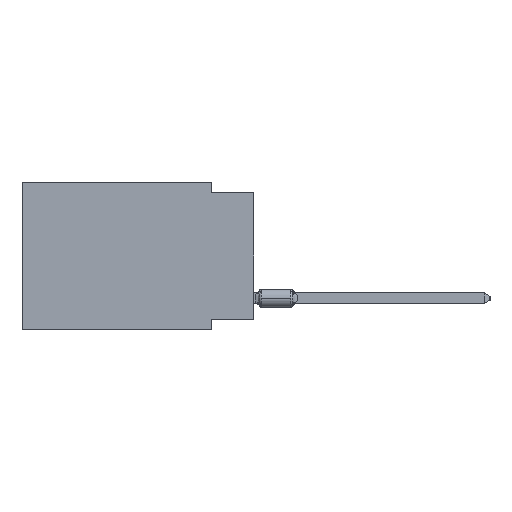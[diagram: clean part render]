
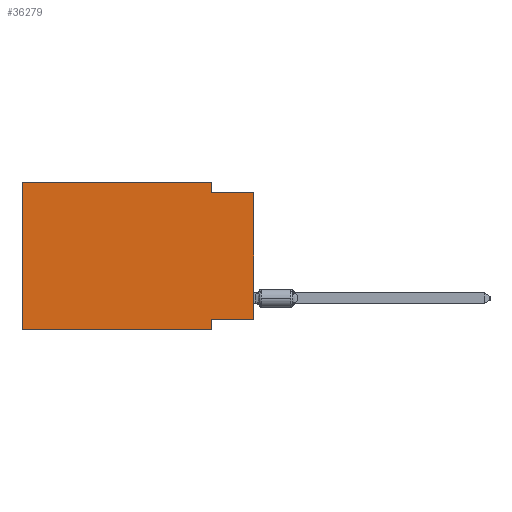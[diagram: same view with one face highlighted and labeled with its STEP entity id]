
A CAD part, left-side view. The second image highlights one B-rep face of the part: STEP entity #36279.
In plain terms, the highlighted planar face has unit normal (-1, 0, 0).
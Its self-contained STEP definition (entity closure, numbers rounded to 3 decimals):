
#119 = VERTEX_POINT ( 'NONE', #2763 ) ;
#2763 = CARTESIAN_POINT ( 'NONE',  ( 0., 0., -0.635 ) ) ;
#3235 = DIRECTION ( 'NONE',  ( 0., 0., -1. ) ) ;
#4117 = EDGE_LOOP ( 'NONE', ( #35548, #5584, #42937, #17807, #14071, #9542, #34353, #60450 ) ) ;
#5584 = ORIENTED_EDGE ( 'NONE', *, *, #37169, .F. ) ;
#5934 = EDGE_CURVE ( 'NONE', #43133, #39119, #27997, .T. ) ;
#6239 = DIRECTION ( 'NONE',  ( 0., 0., -1. ) ) ;
#9410 = CARTESIAN_POINT ( 'NONE',  ( 0., 0., -0.635 ) ) ;
#9542 = ORIENTED_EDGE ( 'NONE', *, *, #14553, .T. ) ;
#9962 = CARTESIAN_POINT ( 'NONE',  ( 0., 2.54, -8.89 ) ) ;
#11250 = EDGE_CURVE ( 'NONE', #32116, #18363, #16929, .T. ) ;
#12801 = LINE ( 'NONE', #58057, #47724 ) ;
#13343 = VECTOR ( 'NONE', #50276, 1000. ) ;
#13557 = CARTESIAN_POINT ( 'NONE',  ( 0., 0., 0. ) ) ;
#14071 = ORIENTED_EDGE ( 'NONE', *, *, #25599, .F. ) ;
#14552 = EDGE_CURVE ( 'NONE', #55181, #43133, #42633, .T. ) ;
#14553 = EDGE_CURVE ( 'NONE', #52668, #39119, #12801, .T. ) ;
#15044 = VERTEX_POINT ( 'NONE', #65896 ) ;
#15582 = DIRECTION ( 'NONE',  ( 0., -1., 0. ) ) ;
#15606 = CARTESIAN_POINT ( 'NONE',  ( 0., 13.97, 0. ) ) ;
#15984 = CARTESIAN_POINT ( 'NONE',  ( 0., 13.97, -8.89 ) ) ;
#16929 = LINE ( 'NONE', #57117, #32574 ) ;
#17807 = ORIENTED_EDGE ( 'NONE', *, *, #11250, .F. ) ;
#18363 = VERTEX_POINT ( 'NONE', #46638 ) ;
#18492 = CARTESIAN_POINT ( 'NONE',  ( 0., 13.97, 0. ) ) ;
#18767 = CARTESIAN_POINT ( 'NONE',  ( 0., 0., -8.255 ) ) ;
#19612 = DIRECTION ( 'NONE',  ( 1., 0., 0. ) ) ;
#20269 = CARTESIAN_POINT ( 'NONE',  ( 0., 13.97, 0. ) ) ;
#21074 = VECTOR ( 'NONE', #33982, 1000. ) ;
#22851 = CARTESIAN_POINT ( 'NONE',  ( 0., 0., -8.255 ) ) ;
#23601 = LINE ( 'NONE', #13557, #21074 ) ;
#25599 = EDGE_CURVE ( 'NONE', #52668, #32116, #43958, .T. ) ;
#27997 = LINE ( 'NONE', #37724, #56881 ) ;
#32116 = VERTEX_POINT ( 'NONE', #15606 ) ;
#32574 = VECTOR ( 'NONE', #15582, 1000. ) ;
#33060 = LINE ( 'NONE', #53506, #38895 ) ;
#33420 = CARTESIAN_POINT ( 'NONE',  ( 0., 2.54, -8.255 ) ) ;
#33758 = VECTOR ( 'NONE', #58721, 1000. ) ;
#33982 = DIRECTION ( 'NONE',  ( 0., 0., 1. ) ) ;
#34353 = ORIENTED_EDGE ( 'NONE', *, *, #5934, .F. ) ;
#34866 = LINE ( 'NONE', #9410, #13343 ) ;
#35548 = ORIENTED_EDGE ( 'NONE', *, *, #62604, .T. ) ;
#36279 = ADVANCED_FACE ( 'NONE', ( #41028 ), #55794, .F. ) ;
#37169 = EDGE_CURVE ( 'NONE', #15044, #119, #34866, .T. ) ;
#37724 = CARTESIAN_POINT ( 'NONE',  ( 0., 2.54, -8.89 ) ) ;
#38595 = DIRECTION ( 'NONE',  ( 0., -1., 0. ) ) ;
#38895 = VECTOR ( 'NONE', #3235, 1000. ) ;
#39119 = VERTEX_POINT ( 'NONE', #9962 ) ;
#40052 = DIRECTION ( 'NONE',  ( 0., 0., -1. ) ) ;
#41028 = FACE_OUTER_BOUND ( 'NONE', #4117, .T. ) ;
#42120 = AXIS2_PLACEMENT_3D ( 'NONE', #20269, #19612, #40052 ) ;
#42633 = LINE ( 'NONE', #22851, #33758 ) ;
#42937 = ORIENTED_EDGE ( 'NONE', *, *, #64517, .F. ) ;
#43133 = VERTEX_POINT ( 'NONE', #33420 ) ;
#43958 = LINE ( 'NONE', #18492, #44962 ) ;
#44962 = VECTOR ( 'NONE', #59378, 1000. ) ;
#46638 = CARTESIAN_POINT ( 'NONE',  ( 0., 2.54, 0. ) ) ;
#47724 = VECTOR ( 'NONE', #38595, 1000. ) ;
#50276 = DIRECTION ( 'NONE',  ( 0., -1., 0. ) ) ;
#52668 = VERTEX_POINT ( 'NONE', #15984 ) ;
#53506 = CARTESIAN_POINT ( 'NONE',  ( 0., 2.54, 0. ) ) ;
#55181 = VERTEX_POINT ( 'NONE', #18767 ) ;
#55794 = PLANE ( 'NONE',  #42120 ) ;
#56881 = VECTOR ( 'NONE', #6239, 1000. ) ;
#57117 = CARTESIAN_POINT ( 'NONE',  ( 0., 13.97, 0. ) ) ;
#58057 = CARTESIAN_POINT ( 'NONE',  ( 0., 13.97, -8.89 ) ) ;
#58721 = DIRECTION ( 'NONE',  ( 0., 1., 0. ) ) ;
#59378 = DIRECTION ( 'NONE',  ( 0., 0., 1. ) ) ;
#60450 = ORIENTED_EDGE ( 'NONE', *, *, #14552, .F. ) ;
#62604 = EDGE_CURVE ( 'NONE', #55181, #119, #23601, .T. ) ;
#64517 = EDGE_CURVE ( 'NONE', #18363, #15044, #33060, .T. ) ;
#65896 = CARTESIAN_POINT ( 'NONE',  ( 0., 2.54, -0.635 ) ) ;
